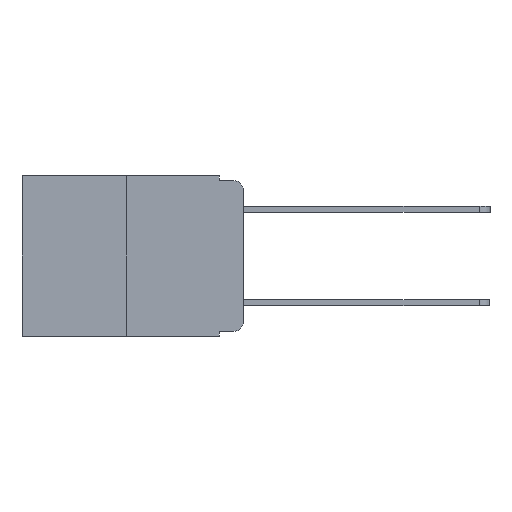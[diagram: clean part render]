
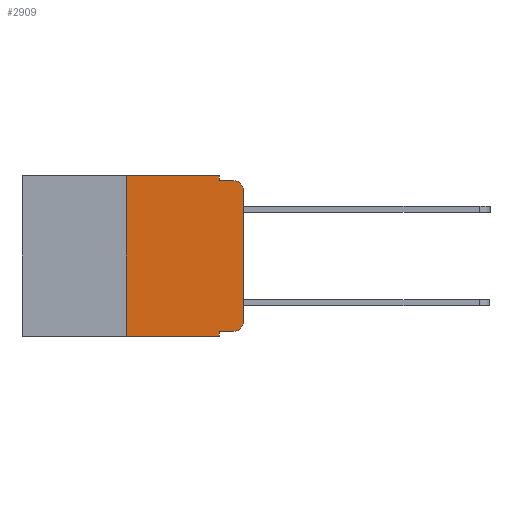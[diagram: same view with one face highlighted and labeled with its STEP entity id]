
A CAD part, left-side view. The second image highlights one B-rep face of the part: STEP entity #2909.
In plain terms, the highlighted planar face has unit normal (-1, 0, 0).
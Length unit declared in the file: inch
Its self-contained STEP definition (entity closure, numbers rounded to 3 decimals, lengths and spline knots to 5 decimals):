
#643 = ORIENTED_EDGE ( 'NONE', *, *, #6636, .T. ) ;
#744 = VERTEX_POINT ( 'NONE', #10728 ) ;
#791 = EDGE_CURVE ( 'NONE', #9353, #17434, #4522, .T. ) ;
#1495 = ORIENTED_EDGE ( 'NONE', *, *, #19443, .T. ) ;
#1715 = CARTESIAN_POINT ( 'NONE',  ( 0., 0.051, -0.01 ) ) ;
#1866 = CIRCLE ( 'NONE', #4464, 0.02 ) ;
#1918 = LINE ( 'NONE', #1715, #10183 ) ;
#2590 = ORIENTED_EDGE ( 'NONE', *, *, #5575, .T. ) ;
#2678 = CARTESIAN_POINT ( 'NONE',  ( 0., 0.051, -0.333 ) ) ;
#2750 = ORIENTED_EDGE ( 'NONE', *, *, #4466, .F. ) ;
#2899 = VECTOR ( 'NONE', #12547, 39.37008 ) ;
#2909 = ADVANCED_FACE ( 'NONE', ( #4402 ), #16054, .F. ) ;
#3022 = VERTEX_POINT ( 'NONE', #7325 ) ;
#3317 = EDGE_CURVE ( 'NONE', #3022, #13047, #12998, .T. ) ;
#3352 = ORIENTED_EDGE ( 'NONE', *, *, #9404, .T. ) ;
#3575 = DIRECTION ( 'NONE',  ( 0., -1., 0. ) ) ;
#4096 = CARTESIAN_POINT ( 'NONE',  ( 0., 0.02, -0.313 ) ) ;
#4402 = FACE_OUTER_BOUND ( 'NONE', #18948, .T. ) ;
#4464 = AXIS2_PLACEMENT_3D ( 'NONE', #7983, #18772, #9565 ) ;
#4466 = EDGE_CURVE ( 'NONE', #13047, #744, #1918, .T. ) ;
#4522 = LINE ( 'NONE', #10537, #16939 ) ;
#5149 = LINE ( 'NONE', #19209, #12502 ) ;
#5390 = VECTOR ( 'NONE', #20283, 39.37008 ) ;
#5575 = EDGE_CURVE ( 'NONE', #11025, #744, #1866, .T. ) ;
#5752 = DIRECTION ( 'NONE',  ( 0., 0., -1. ) ) ;
#5898 = LINE ( 'NONE', #18763, #5390 ) ;
#6091 = DIRECTION ( 'NONE',  ( 0., -1., 0. ) ) ;
#6510 = EDGE_CURVE ( 'NONE', #17434, #3022, #5149, .T. ) ;
#6540 = CARTESIAN_POINT ( 'NONE',  ( 0., 0.25, 0. ) ) ;
#6636 = EDGE_CURVE ( 'NONE', #18953, #11025, #14710, .T. ) ;
#6933 = CARTESIAN_POINT ( 'NONE',  ( 0., 0.051, -0.01 ) ) ;
#7246 = CARTESIAN_POINT ( 'NONE',  ( 0., 0., -0.313 ) ) ;
#7325 = CARTESIAN_POINT ( 'NONE',  ( 0., 0.051, 0. ) ) ;
#7983 = CARTESIAN_POINT ( 'NONE',  ( 0., 0.02, -0.03 ) ) ;
#8149 = DIRECTION ( 'NONE',  ( 0., 0., -1. ) ) ;
#8625 = VECTOR ( 'NONE', #6091, 39.37008 ) ;
#8954 = AXIS2_PLACEMENT_3D ( 'NONE', #17579, #19143, #9958 ) ;
#9353 = VERTEX_POINT ( 'NONE', #15495 ) ;
#9359 = VECTOR ( 'NONE', #8149, 39.37008 ) ;
#9404 = EDGE_CURVE ( 'NONE', #9353, #9818, #11931, .T. ) ;
#9565 = DIRECTION ( 'NONE',  ( 0., 0., -1. ) ) ;
#9635 = CARTESIAN_POINT ( 'NONE',  ( 0., 0.02, -0.333 ) ) ;
#9818 = VERTEX_POINT ( 'NONE', #10458 ) ;
#9958 = DIRECTION ( 'NONE',  ( 0., 0., -1. ) ) ;
#10183 = VECTOR ( 'NONE', #3575, 39.37008 ) ;
#10458 = CARTESIAN_POINT ( 'NONE',  ( 0., 0.051, -0.343 ) ) ;
#10537 = CARTESIAN_POINT ( 'NONE',  ( 0., 0.25, 0. ) ) ;
#10717 = ORIENTED_EDGE ( 'NONE', *, *, #6510, .F. ) ;
#10728 = CARTESIAN_POINT ( 'NONE',  ( 0., 0.02, -0.01 ) ) ;
#10993 = CARTESIAN_POINT ( 'NONE',  ( 0., 0.473, -0.343 ) ) ;
#11025 = VERTEX_POINT ( 'NONE', #11485 ) ;
#11374 = CIRCLE ( 'NONE', #15508, 0.02 ) ;
#11485 = CARTESIAN_POINT ( 'NONE',  ( 0., 0., -0.03 ) ) ;
#11931 = LINE ( 'NONE', #10993, #2899 ) ;
#12502 = VECTOR ( 'NONE', #20715, 39.37008 ) ;
#12547 = DIRECTION ( 'NONE',  ( 0., -1., 0. ) ) ;
#12998 = LINE ( 'NONE', #17376, #9359 ) ;
#13047 = VERTEX_POINT ( 'NONE', #6933 ) ;
#13681 = VERTEX_POINT ( 'NONE', #16111 ) ;
#13753 = ORIENTED_EDGE ( 'NONE', *, *, #3317, .F. ) ;
#14181 = VERTEX_POINT ( 'NONE', #9635 ) ;
#14710 = LINE ( 'NONE', #17919, #18715 ) ;
#15090 = DIRECTION ( 'NONE',  ( -1., 0., 0. ) ) ;
#15495 = CARTESIAN_POINT ( 'NONE',  ( 0., 0.25, -0.343 ) ) ;
#15508 = AXIS2_PLACEMENT_3D ( 'NONE', #4096, #15090, #5752 ) ;
#16054 = PLANE ( 'NONE',  #8954 ) ;
#16111 = CARTESIAN_POINT ( 'NONE',  ( 0., 0.051, -0.333 ) ) ;
#16129 = ORIENTED_EDGE ( 'NONE', *, *, #20446, .F. ) ;
#16814 = LINE ( 'NONE', #2678, #8625 ) ;
#16939 = VECTOR ( 'NONE', #19916, 39.37008 ) ;
#17376 = CARTESIAN_POINT ( 'NONE',  ( 0., 0.051, 0. ) ) ;
#17434 = VERTEX_POINT ( 'NONE', #6540 ) ;
#17579 = CARTESIAN_POINT ( 'NONE',  ( 0., 0.473, 0. ) ) ;
#17812 = ORIENTED_EDGE ( 'NONE', *, *, #18403, .T. ) ;
#17919 = CARTESIAN_POINT ( 'NONE',  ( 0., 0., 0. ) ) ;
#18403 = EDGE_CURVE ( 'NONE', #14181, #18953, #11374, .T. ) ;
#18715 = VECTOR ( 'NONE', #19471, 39.37008 ) ;
#18763 = CARTESIAN_POINT ( 'NONE',  ( 0., 0.051, 0. ) ) ;
#18772 = DIRECTION ( 'NONE',  ( -1., 0., 0. ) ) ;
#18928 = ORIENTED_EDGE ( 'NONE', *, *, #791, .F. ) ;
#18948 = EDGE_LOOP ( 'NONE', ( #643, #2590, #2750, #13753, #10717, #18928, #3352, #16129, #1495, #17812 ) ) ;
#18953 = VERTEX_POINT ( 'NONE', #7246 ) ;
#19143 = DIRECTION ( 'NONE',  ( 1., 0., 0. ) ) ;
#19209 = CARTESIAN_POINT ( 'NONE',  ( 0., 0.473, 0. ) ) ;
#19443 = EDGE_CURVE ( 'NONE', #13681, #14181, #16814, .T. ) ;
#19471 = DIRECTION ( 'NONE',  ( 0., 0., 1. ) ) ;
#19916 = DIRECTION ( 'NONE',  ( 0., 0., 1. ) ) ;
#20283 = DIRECTION ( 'NONE',  ( 0., 0., -1. ) ) ;
#20446 = EDGE_CURVE ( 'NONE', #13681, #9818, #5898, .T. ) ;
#20715 = DIRECTION ( 'NONE',  ( 0., -1., 0. ) ) ;
